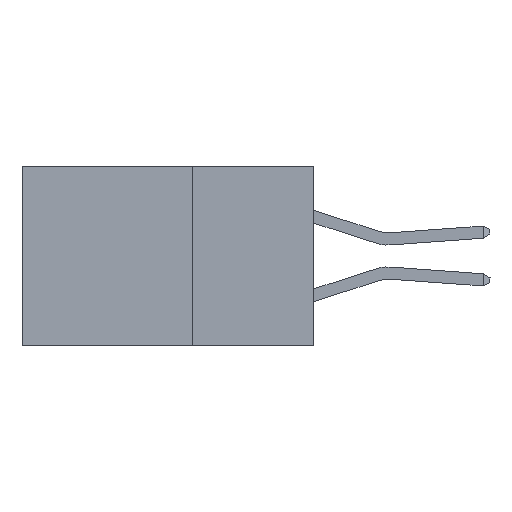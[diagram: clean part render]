
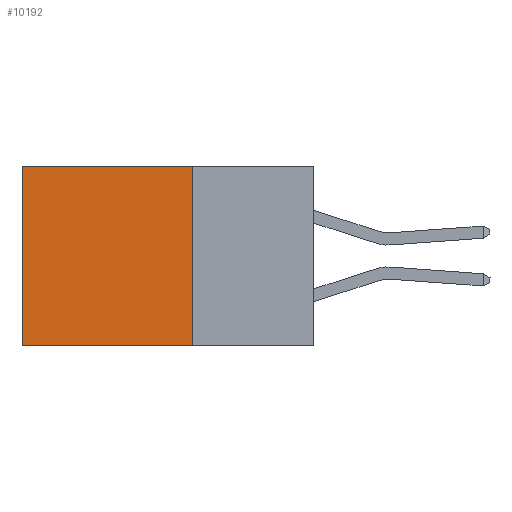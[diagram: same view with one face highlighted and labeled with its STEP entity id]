
A CAD part, left-side view. The second image highlights one B-rep face of the part: STEP entity #10192.
In plain terms, the highlighted planar face has unit normal (-1, 0, 0).
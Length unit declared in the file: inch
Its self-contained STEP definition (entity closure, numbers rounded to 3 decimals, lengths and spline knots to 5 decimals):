
#565 = CARTESIAN_POINT ( 'NONE',  ( 0.2875, 0.6, -0.37 ) ) ;
#662 = EDGE_LOOP ( 'NONE', ( #14201, #12603, #17319, #16484 ) ) ;
#1225 = CARTESIAN_POINT ( 'NONE',  ( 0.2875, 0.25, 0. ) ) ;
#2898 = VECTOR ( 'NONE', #14495, 39.37008 ) ;
#2917 = EDGE_CURVE ( 'NONE', #14435, #13428, #3712, .T. ) ;
#3002 = VECTOR ( 'NONE', #18587, 39.37008 ) ;
#3046 = CARTESIAN_POINT ( 'NONE',  ( 0.2875, 0.25, -0.37 ) ) ;
#3078 = VECTOR ( 'NONE', #7812, 39.37008 ) ;
#3704 = DIRECTION ( 'NONE',  ( 0., 0., -1. ) ) ;
#3712 = LINE ( 'NONE', #1225, #3002 ) ;
#6754 = VERTEX_POINT ( 'NONE', #3046 ) ;
#7265 = CARTESIAN_POINT ( 'NONE',  ( 0.2875, 0.25, -0.37 ) ) ;
#7320 = VECTOR ( 'NONE', #3704, 39.37008 ) ;
#7812 = DIRECTION ( 'NONE',  ( 0., 1., 0. ) ) ;
#7928 = LINE ( 'NONE', #14364, #2898 ) ;
#9813 = VERTEX_POINT ( 'NONE', #565 ) ;
#10029 = LINE ( 'NONE', #18208, #7320 ) ;
#10036 = EDGE_CURVE ( 'NONE', #13428, #9813, #10029, .T. ) ;
#10192 = ADVANCED_FACE ( 'NONE', ( #17462 ), #13498, .F. ) ;
#10219 = CARTESIAN_POINT ( 'NONE',  ( 0.2875, 0.6, 0. ) ) ;
#10519 = CARTESIAN_POINT ( 'NONE',  ( 0.2875, 0.25, 0. ) ) ;
#11236 = AXIS2_PLACEMENT_3D ( 'NONE', #10519, #13431, #16192 ) ;
#11594 = EDGE_CURVE ( 'NONE', #14435, #6754, #7928, .T. ) ;
#12603 = ORIENTED_EDGE ( 'NONE', *, *, #13461, .F. ) ;
#13428 = VERTEX_POINT ( 'NONE', #10219 ) ;
#13431 = DIRECTION ( 'NONE',  ( 1., 0., 0. ) ) ;
#13461 = EDGE_CURVE ( 'NONE', #6754, #9813, #16224, .T. ) ;
#13498 = PLANE ( 'NONE',  #11236 ) ;
#14201 = ORIENTED_EDGE ( 'NONE', *, *, #10036, .T. ) ;
#14364 = CARTESIAN_POINT ( 'NONE',  ( 0.2875, 0.25, 0. ) ) ;
#14435 = VERTEX_POINT ( 'NONE', #17119 ) ;
#14495 = DIRECTION ( 'NONE',  ( 0., 0., -1. ) ) ;
#16192 = DIRECTION ( 'NONE',  ( 0., 0., -1. ) ) ;
#16224 = LINE ( 'NONE', #7265, #3078 ) ;
#16484 = ORIENTED_EDGE ( 'NONE', *, *, #2917, .T. ) ;
#17119 = CARTESIAN_POINT ( 'NONE',  ( 0.2875, 0.25, 0. ) ) ;
#17319 = ORIENTED_EDGE ( 'NONE', *, *, #11594, .F. ) ;
#17462 = FACE_OUTER_BOUND ( 'NONE', #662, .T. ) ;
#18208 = CARTESIAN_POINT ( 'NONE',  ( 0.2875, 0.6, 0. ) ) ;
#18587 = DIRECTION ( 'NONE',  ( 0., 1., 0. ) ) ;
